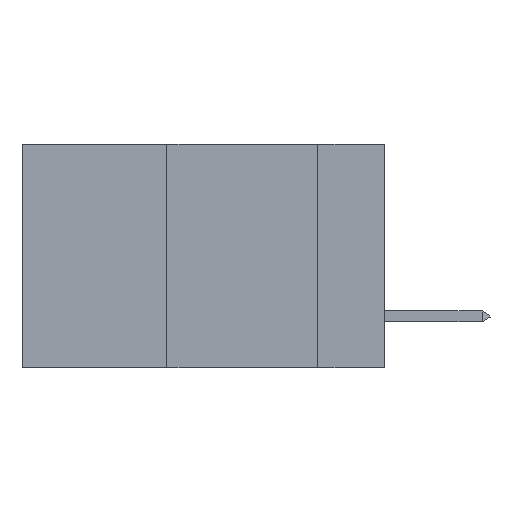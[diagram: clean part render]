
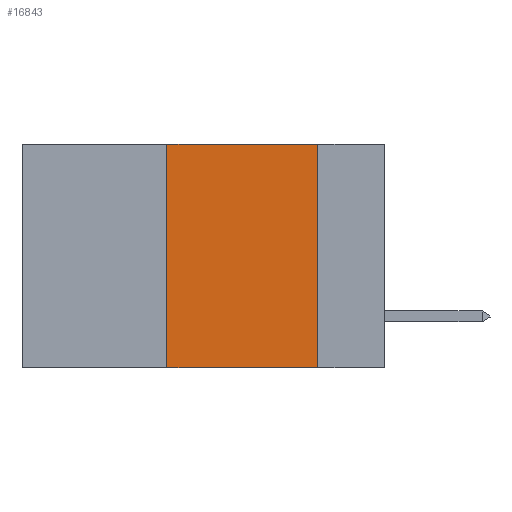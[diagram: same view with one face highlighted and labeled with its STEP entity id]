
A CAD part, left-side view. The second image highlights one B-rep face of the part: STEP entity #16843.
In plain terms, the highlighted planar face has unit normal (-1, 0, 0).
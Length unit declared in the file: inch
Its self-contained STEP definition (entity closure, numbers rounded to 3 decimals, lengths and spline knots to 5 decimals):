
#133 = EDGE_CURVE ( 'NONE', #7344, #12274, #14477, .T. ) ;
#609 = LINE ( 'NONE', #14138, #15936 ) ;
#973 = DIRECTION ( 'NONE',  ( 1., 0., 0. ) ) ;
#1050 = EDGE_CURVE ( 'NONE', #15062, #14207, #609, .T. ) ;
#1108 = CARTESIAN_POINT ( 'NONE',  ( 0., 0.36, 0. ) ) ;
#1371 = FACE_OUTER_BOUND ( 'NONE', #17472, .T. ) ;
#2870 = DIRECTION ( 'NONE',  ( 0., -1., 0. ) ) ;
#4113 = CARTESIAN_POINT ( 'NONE',  ( 0., 0.11, 0. ) ) ;
#4430 = ORIENTED_EDGE ( 'NONE', *, *, #10736, .F. ) ;
#5141 = CARTESIAN_POINT ( 'NONE',  ( 0., 0.6, 0. ) ) ;
#6057 = CARTESIAN_POINT ( 'NONE',  ( 0., 0.11, -0.37 ) ) ;
#6234 = EDGE_CURVE ( 'NONE', #15062, #12274, #13507, .T. ) ;
#6623 = VECTOR ( 'NONE', #16114, 39.37008 ) ;
#7153 = CARTESIAN_POINT ( 'NONE',  ( 0., 0.11, 0. ) ) ;
#7287 = ORIENTED_EDGE ( 'NONE', *, *, #133, .F. ) ;
#7334 = DIRECTION ( 'NONE',  ( 0., 0., 1. ) ) ;
#7344 = VERTEX_POINT ( 'NONE', #7153 ) ;
#7808 = ORIENTED_EDGE ( 'NONE', *, *, #1050, .F. ) ;
#8466 = AXIS2_PLACEMENT_3D ( 'NONE', #5141, #973, #9132 ) ;
#8835 = DIRECTION ( 'NONE',  ( 0., -1., 0. ) ) ;
#9057 = VECTOR ( 'NONE', #8835, 39.37008 ) ;
#9132 = DIRECTION ( 'NONE',  ( 0., 0., -1. ) ) ;
#9190 = PLANE ( 'NONE',  #8466 ) ;
#9704 = CARTESIAN_POINT ( 'NONE',  ( 0., 0.36, -0.37 ) ) ;
#10736 = EDGE_CURVE ( 'NONE', #14207, #7344, #13255, .T. ) ;
#10995 = CARTESIAN_POINT ( 'NONE',  ( 0., 0.6, 0. ) ) ;
#12274 = VERTEX_POINT ( 'NONE', #6057 ) ;
#12792 = CARTESIAN_POINT ( 'NONE',  ( 0., 0.6, -0.37 ) ) ;
#13255 = LINE ( 'NONE', #10995, #16678 ) ;
#13507 = LINE ( 'NONE', #12792, #9057 ) ;
#14138 = CARTESIAN_POINT ( 'NONE',  ( 0., 0.36, 0. ) ) ;
#14207 = VERTEX_POINT ( 'NONE', #1108 ) ;
#14477 = LINE ( 'NONE', #4113, #6623 ) ;
#15062 = VERTEX_POINT ( 'NONE', #9704 ) ;
#15163 = ORIENTED_EDGE ( 'NONE', *, *, #6234, .T. ) ;
#15936 = VECTOR ( 'NONE', #7334, 39.37008 ) ;
#16114 = DIRECTION ( 'NONE',  ( 0., 0., -1. ) ) ;
#16678 = VECTOR ( 'NONE', #2870, 39.37008 ) ;
#16843 = ADVANCED_FACE ( 'NONE', ( #1371 ), #9190, .F. ) ;
#17472 = EDGE_LOOP ( 'NONE', ( #7287, #4430, #7808, #15163 ) ) ;
